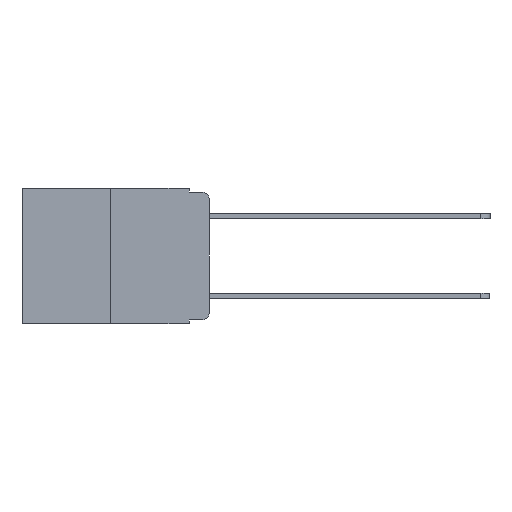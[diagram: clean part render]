
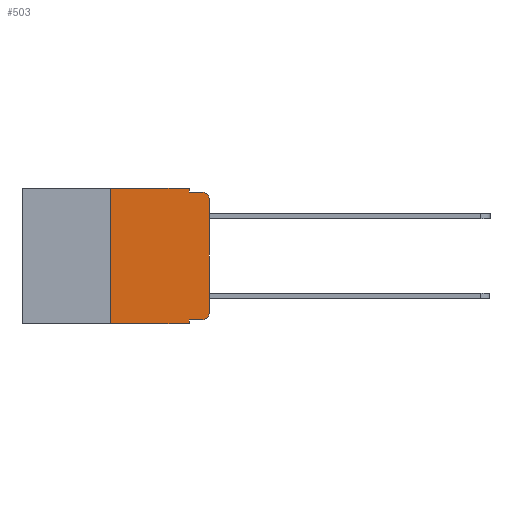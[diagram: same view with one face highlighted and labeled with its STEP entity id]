
A CAD part, left-side view. The second image highlights one B-rep face of the part: STEP entity #503.
In plain terms, the highlighted planar face has unit normal (-1, 0, 0).
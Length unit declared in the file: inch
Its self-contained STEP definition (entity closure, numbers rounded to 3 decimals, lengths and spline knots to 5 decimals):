
#60 = ORIENTED_EDGE ( 'NONE', *, *, #1301, .F. ) ;
#101 = VERTEX_POINT ( 'NONE', #6728 ) ;
#271 = ORIENTED_EDGE ( 'NONE', *, *, #8892, .T. ) ;
#319 = EDGE_LOOP ( 'NONE', ( #2490, #7107, #10269, #1514, #60, #9519, #2888, #1435, #9714, #271 ) ) ;
#443 = CARTESIAN_POINT ( 'NONE',  ( 0., 0.051, 0. ) ) ;
#491 = DIRECTION ( 'NONE',  ( 0., -1., 0. ) ) ;
#503 = ADVANCED_FACE ( 'NONE', ( #1103 ), #7732, .F. ) ;
#562 = EDGE_CURVE ( 'NONE', #8929, #6244, #7508, .T. ) ;
#804 = LINE ( 'NONE', #10125, #6073 ) ;
#1031 = CARTESIAN_POINT ( 'NONE',  ( 0., 0.051, -0.333 ) ) ;
#1103 = FACE_OUTER_BOUND ( 'NONE', #319, .T. ) ;
#1136 = CARTESIAN_POINT ( 'NONE',  ( 0., 0.051, -0.343 ) ) ;
#1301 = EDGE_CURVE ( 'NONE', #8442, #5765, #4035, .T. ) ;
#1435 = ORIENTED_EDGE ( 'NONE', *, *, #562, .F. ) ;
#1445 = CARTESIAN_POINT ( 'NONE',  ( 0., 0.25, -0.343 ) ) ;
#1514 = ORIENTED_EDGE ( 'NONE', *, *, #4182, .F. ) ;
#1723 = EDGE_CURVE ( 'NONE', #4218, #6244, #10619, .T. ) ;
#1984 = VECTOR ( 'NONE', #8264, 39.37008 ) ;
#2034 = CIRCLE ( 'NONE', #5268, 0.02 ) ;
#2363 = CARTESIAN_POINT ( 'NONE',  ( 0., 0.051, -0.01 ) ) ;
#2471 = DIRECTION ( 'NONE',  ( -1., 0., 0. ) ) ;
#2490 = ORIENTED_EDGE ( 'NONE', *, *, #6521, .T. ) ;
#2888 = ORIENTED_EDGE ( 'NONE', *, *, #1723, .T. ) ;
#2964 = CARTESIAN_POINT ( 'NONE',  ( 0., 0.473, 0. ) ) ;
#3211 = CARTESIAN_POINT ( 'NONE',  ( 0., 0.051, -0.333 ) ) ;
#3266 = DIRECTION ( 'NONE',  ( 0., -1., 0. ) ) ;
#3673 = DIRECTION ( 'NONE',  ( 1., 0., 0. ) ) ;
#3701 = CARTESIAN_POINT ( 'NONE',  ( 0., 0., -0.313 ) ) ;
#3961 = VERTEX_POINT ( 'NONE', #3701 ) ;
#4035 = LINE ( 'NONE', #2964, #10381 ) ;
#4182 = EDGE_CURVE ( 'NONE', #5765, #5157, #6669, .T. ) ;
#4218 = VERTEX_POINT ( 'NONE', #1445 ) ;
#4371 = AXIS2_PLACEMENT_3D ( 'NONE', #5906, #3673, #9126 ) ;
#4537 = DIRECTION ( 'NONE',  ( -1., 0., 0. ) ) ;
#4826 = VERTEX_POINT ( 'NONE', #7587 ) ;
#4865 = CARTESIAN_POINT ( 'NONE',  ( 0., 0.25, 0. ) ) ;
#5087 = CARTESIAN_POINT ( 'NONE',  ( 0., 0.02, -0.01 ) ) ;
#5157 = VERTEX_POINT ( 'NONE', #8142 ) ;
#5268 = AXIS2_PLACEMENT_3D ( 'NONE', #9521, #4537, #10321 ) ;
#5363 = EDGE_CURVE ( 'NONE', #5157, #10942, #5708, .T. ) ;
#5432 = VECTOR ( 'NONE', #3266, 39.37008 ) ;
#5708 = LINE ( 'NONE', #2363, #5432 ) ;
#5765 = VERTEX_POINT ( 'NONE', #9806 ) ;
#5814 = VECTOR ( 'NONE', #10153, 39.37008 ) ;
#5906 = CARTESIAN_POINT ( 'NONE',  ( 0., 0.473, 0. ) ) ;
#5935 = EDGE_CURVE ( 'NONE', #4826, #10942, #7133, .T. ) ;
#6008 = CARTESIAN_POINT ( 'NONE',  ( 0., 0.051, 0. ) ) ;
#6073 = VECTOR ( 'NONE', #6910, 39.37008 ) ;
#6244 = VERTEX_POINT ( 'NONE', #1136 ) ;
#6292 = DIRECTION ( 'NONE',  ( 0., 0., -1. ) ) ;
#6521 = EDGE_CURVE ( 'NONE', #3961, #4826, #804, .T. ) ;
#6669 = LINE ( 'NONE', #443, #1984 ) ;
#6678 = DIRECTION ( 'NONE',  ( 0., -1., 0. ) ) ;
#6728 = CARTESIAN_POINT ( 'NONE',  ( 0., 0.02, -0.333 ) ) ;
#6733 = AXIS2_PLACEMENT_3D ( 'NONE', #7635, #2471, #8451 ) ;
#6910 = DIRECTION ( 'NONE',  ( 0., 0., 1. ) ) ;
#7092 = VECTOR ( 'NONE', #6678, 39.37008 ) ;
#7107 = ORIENTED_EDGE ( 'NONE', *, *, #5935, .T. ) ;
#7133 = CIRCLE ( 'NONE', #6733, 0.02 ) ;
#7508 = LINE ( 'NONE', #6008, #9667 ) ;
#7587 = CARTESIAN_POINT ( 'NONE',  ( 0., 0., -0.03 ) ) ;
#7635 = CARTESIAN_POINT ( 'NONE',  ( 0., 0.02, -0.03 ) ) ;
#7732 = PLANE ( 'NONE',  #4371 ) ;
#7806 = EDGE_CURVE ( 'NONE', #8929, #101, #9249, .T. ) ;
#8142 = CARTESIAN_POINT ( 'NONE',  ( 0., 0.051, -0.01 ) ) ;
#8264 = DIRECTION ( 'NONE',  ( 0., 0., -1. ) ) ;
#8423 = CARTESIAN_POINT ( 'NONE',  ( 0., 0.473, -0.343 ) ) ;
#8442 = VERTEX_POINT ( 'NONE', #4865 ) ;
#8451 = DIRECTION ( 'NONE',  ( 0., 0., -1. ) ) ;
#8495 = VECTOR ( 'NONE', #9456, 39.37008 ) ;
#8892 = EDGE_CURVE ( 'NONE', #101, #3961, #2034, .T. ) ;
#8929 = VERTEX_POINT ( 'NONE', #1031 ) ;
#9126 = DIRECTION ( 'NONE',  ( 0., 0., -1. ) ) ;
#9249 = LINE ( 'NONE', #3211, #7092 ) ;
#9348 = CARTESIAN_POINT ( 'NONE',  ( 0., 0.25, 0. ) ) ;
#9456 = DIRECTION ( 'NONE',  ( 0., -1., 0. ) ) ;
#9519 = ORIENTED_EDGE ( 'NONE', *, *, #11022, .F. ) ;
#9521 = CARTESIAN_POINT ( 'NONE',  ( 0., 0.02, -0.313 ) ) ;
#9667 = VECTOR ( 'NONE', #6292, 39.37008 ) ;
#9714 = ORIENTED_EDGE ( 'NONE', *, *, #7806, .T. ) ;
#9806 = CARTESIAN_POINT ( 'NONE',  ( 0., 0.051, 0. ) ) ;
#10125 = CARTESIAN_POINT ( 'NONE',  ( 0., 0., 0. ) ) ;
#10153 = DIRECTION ( 'NONE',  ( 0., 0., 1. ) ) ;
#10156 = LINE ( 'NONE', #9348, #5814 ) ;
#10269 = ORIENTED_EDGE ( 'NONE', *, *, #5363, .F. ) ;
#10321 = DIRECTION ( 'NONE',  ( 0., 0., -1. ) ) ;
#10381 = VECTOR ( 'NONE', #491, 39.37008 ) ;
#10619 = LINE ( 'NONE', #8423, #8495 ) ;
#10942 = VERTEX_POINT ( 'NONE', #5087 ) ;
#11022 = EDGE_CURVE ( 'NONE', #4218, #8442, #10156, .T. ) ;
